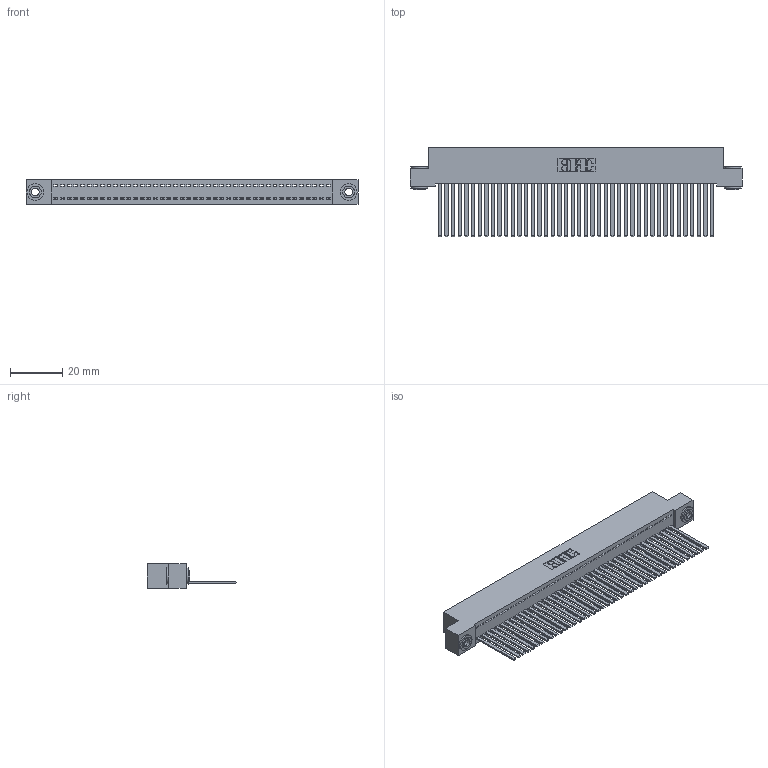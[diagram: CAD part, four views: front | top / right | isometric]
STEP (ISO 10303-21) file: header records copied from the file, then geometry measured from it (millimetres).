
FILE_DESCRIPTION (( 'STEP AP203' ), '1' );
FILE_NAME ('342-042-544-103.STEP', '2018-08-12T13:13:44', ( '' ), ( '' ), 'SwSTEP 2.0', 'SolidWorks 2016', '' );
FILE_SCHEMA (( 'CONFIG_CONTROL_DESIGN' ));
Length unit declared in the file: inch
Products named in the file (4): 342 Part_.156 TH; 345-292-001_345-293-144; 342-250-002_345-250-002-102; 342-042-544-103
Assembly tree (45 placements, depth 2):
  342-042-544-103
    342 Part_.156 TH
    345-292-001_345-293-144  x42
    342-250-002_345-250-002-102  x2
Bounding box: 127 x 34.3 x 9.4 mm (x, y, z)
Volume: 11644.6 mm3; surface area: 18710.1 mm2
Topology: 45 solids, 45 shells, 2332 faces, 7011 edges, 4614 vertices
Faces by surface type: plane 1672, cylinder 652, cone 8
Entity records: 26010 total; most frequent: CARTESIAN_POINT 4463, ORIENTED_EDGE 4434, DIRECTION 3795, EDGE_CURVE 2217, VECTOR 2069, LINE 2069, VERTEX_POINT 1474, AXIS2_PLACEMENT_3D 863
